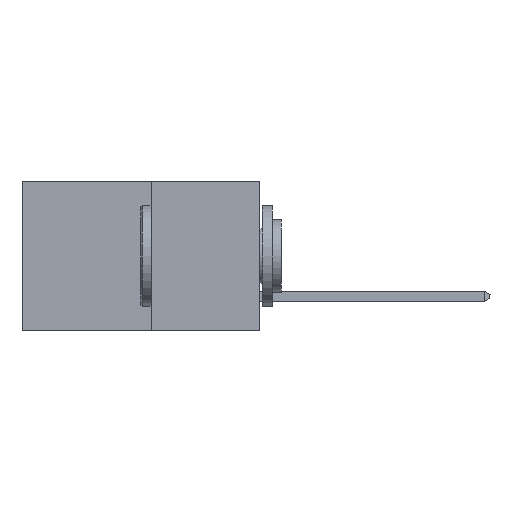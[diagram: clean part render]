
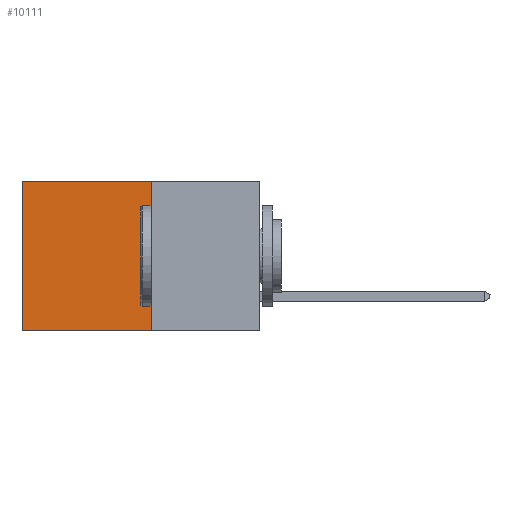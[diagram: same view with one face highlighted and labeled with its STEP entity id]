
A CAD part, left-side view. The second image highlights one B-rep face of the part: STEP entity #10111.
In plain terms, the highlighted planar face has unit normal (-1, 0, 0).
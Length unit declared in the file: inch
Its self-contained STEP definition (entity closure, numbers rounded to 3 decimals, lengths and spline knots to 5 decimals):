
#73 = VERTEX_POINT ( 'NONE', #2360 ) ;
#507 = LINE ( 'NONE', #12266, #9733 ) ;
#1161 = FACE_OUTER_BOUND ( 'NONE', #12911, .T. ) ;
#1176 = VECTOR ( 'NONE', #10621, 39.37008 ) ;
#1206 = AXIS2_PLACEMENT_3D ( 'NONE', #3915, #5093, #12568 ) ;
#1223 = VERTEX_POINT ( 'NONE', #6934 ) ;
#1588 = CARTESIAN_POINT ( 'NONE',  ( 0.277, 0.27, -0.37 ) ) ;
#1604 = DIRECTION ( 'NONE',  ( 0., 1., 0. ) ) ;
#2298 = ORIENTED_EDGE ( 'NONE', *, *, #5015, .F. ) ;
#2360 = CARTESIAN_POINT ( 'NONE',  ( 0.277, 0.27, 0. ) ) ;
#2802 = CARTESIAN_POINT ( 'NONE',  ( 0.277, 0.27, -0.37 ) ) ;
#3915 = CARTESIAN_POINT ( 'NONE',  ( 0.277, 0.27, -0.37 ) ) ;
#4119 = EDGE_CURVE ( 'NONE', #13258, #13418, #8155, .T. ) ;
#5015 = EDGE_CURVE ( 'NONE', #73, #13258, #507, .T. ) ;
#5093 = DIRECTION ( 'NONE',  ( 1., 0., 0. ) ) ;
#5542 = VECTOR ( 'NONE', #5655, 39.37008 ) ;
#5655 = DIRECTION ( 'NONE',  ( 0., 1., 0. ) ) ;
#5788 = ORIENTED_EDGE ( 'NONE', *, *, #9728, .T. ) ;
#5890 = LINE ( 'NONE', #11135, #5542 ) ;
#6078 = EDGE_CURVE ( 'NONE', #1223, #13418, #7329, .T. ) ;
#6122 = CARTESIAN_POINT ( 'NONE',  ( 0.277, 0.59, -0.37 ) ) ;
#6934 = CARTESIAN_POINT ( 'NONE',  ( 0.277, 0.59, 0. ) ) ;
#7329 = LINE ( 'NONE', #6122, #1176 ) ;
#7796 = VECTOR ( 'NONE', #1604, 39.37008 ) ;
#8155 = LINE ( 'NONE', #1588, #7796 ) ;
#8760 = CARTESIAN_POINT ( 'NONE',  ( 0.277, 0.59, -0.37 ) ) ;
#9728 = EDGE_CURVE ( 'NONE', #73, #1223, #5890, .T. ) ;
#9733 = VECTOR ( 'NONE', #13211, 39.37008 ) ;
#10111 = ADVANCED_FACE ( 'NONE', ( #1161 ), #11642, .F. ) ;
#10621 = DIRECTION ( 'NONE',  ( 0., 0., -1. ) ) ;
#10673 = ORIENTED_EDGE ( 'NONE', *, *, #6078, .T. ) ;
#10981 = ORIENTED_EDGE ( 'NONE', *, *, #4119, .F. ) ;
#11135 = CARTESIAN_POINT ( 'NONE',  ( 0.277, 0.27, 0. ) ) ;
#11642 = PLANE ( 'NONE',  #1206 ) ;
#12266 = CARTESIAN_POINT ( 'NONE',  ( 0.277, 0.27, -0.37 ) ) ;
#12568 = DIRECTION ( 'NONE',  ( 0., 0., -1. ) ) ;
#12911 = EDGE_LOOP ( 'NONE', ( #10673, #10981, #2298, #5788 ) ) ;
#13211 = DIRECTION ( 'NONE',  ( 0., 0., -1. ) ) ;
#13258 = VERTEX_POINT ( 'NONE', #2802 ) ;
#13418 = VERTEX_POINT ( 'NONE', #8760 ) ;
